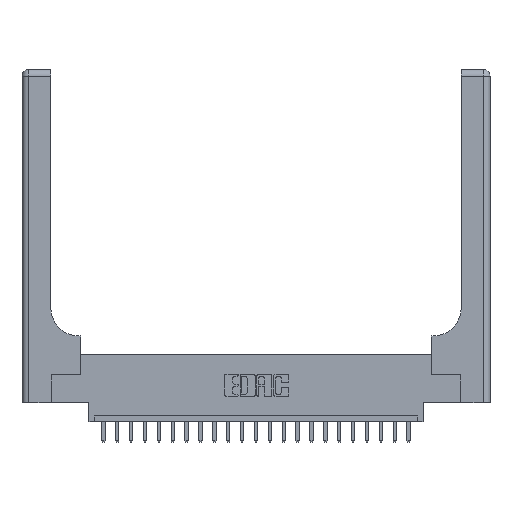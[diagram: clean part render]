
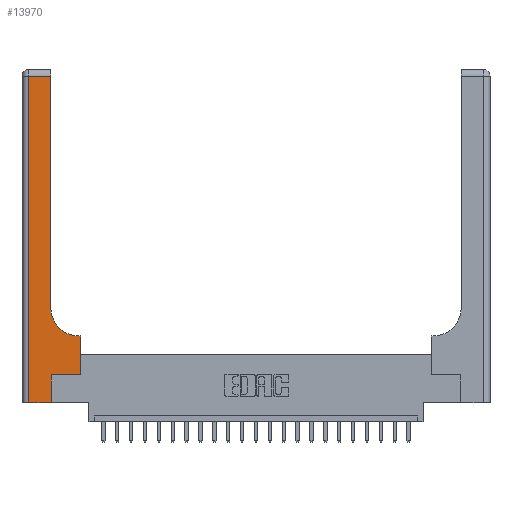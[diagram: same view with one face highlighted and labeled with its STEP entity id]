
A CAD part, top view. The second image highlights one B-rep face of the part: STEP entity #13970.
In plain terms, the highlighted planar face has unit normal (0, 0, 1).
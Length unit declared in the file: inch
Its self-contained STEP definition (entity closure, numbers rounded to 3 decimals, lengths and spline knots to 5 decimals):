
#11 = CARTESIAN_POINT ( 'NONE',  ( 0.26, 0.85, 0.37 ) ) ;
#16 = EDGE_CURVE ( 'NONE', #6308, #11377, #10593, .T. ) ;
#32 = CARTESIAN_POINT ( 'NONE',  ( 0.528, 0.25, 0.37 ) ) ;
#1361 = VECTOR ( 'NONE', #21693, 39.37008 ) ;
#1651 = CARTESIAN_POINT ( 'NONE',  ( 0.26, 2.94, 0.37 ) ) ;
#1661 = LINE ( 'NONE', #3941, #3279 ) ;
#2300 = VERTEX_POINT ( 'NONE', #7074 ) ;
#2553 = LINE ( 'NONE', #12259, #5292 ) ;
#3279 = VECTOR ( 'NONE', #16071, 39.37008 ) ;
#3343 = DIRECTION ( 'NONE',  ( 0., 0., -1. ) ) ;
#3627 = EDGE_CURVE ( 'NONE', #15931, #14777, #4854, .T. ) ;
#3761 = ORIENTED_EDGE ( 'NONE', *, *, #16470, .T. ) ;
#3941 = CARTESIAN_POINT ( 'NONE',  ( 0.26, 3., 0.37 ) ) ;
#4330 = CARTESIAN_POINT ( 'NONE',  ( 0.528, 0.25, 0.37 ) ) ;
#4854 = CIRCLE ( 'NONE', #6995, 0.25 ) ;
#5086 = ORIENTED_EDGE ( 'NONE', *, *, #20870, .T. ) ;
#5292 = VECTOR ( 'NONE', #6880, 39.37008 ) ;
#5703 = ORIENTED_EDGE ( 'NONE', *, *, #12226, .T. ) ;
#5906 = EDGE_CURVE ( 'NONE', #11377, #2300, #9012, .T. ) ;
#6043 = VECTOR ( 'NONE', #6108, 39.37008 ) ;
#6063 = DIRECTION ( 'NONE',  ( -1., 0., 0. ) ) ;
#6108 = DIRECTION ( 'NONE',  ( 1., 0., 0. ) ) ;
#6161 = VERTEX_POINT ( 'NONE', #18413 ) ;
#6300 = VECTOR ( 'NONE', #21127, 39.37008 ) ;
#6308 = VERTEX_POINT ( 'NONE', #6826 ) ;
#6321 = EDGE_LOOP ( 'NONE', ( #7735, #17940, #5086, #5703, #21645, #8040, #14710, #3761, #9540 ) ) ;
#6688 = VERTEX_POINT ( 'NONE', #16374 ) ;
#6826 = CARTESIAN_POINT ( 'NONE',  ( 0.265, 0.25, 0.37 ) ) ;
#6880 = DIRECTION ( 'NONE',  ( -1., 0., 0. ) ) ;
#6995 = AXIS2_PLACEMENT_3D ( 'NONE', #10307, #3343, #11828 ) ;
#7074 = CARTESIAN_POINT ( 'NONE',  ( 0.528, 0.6, 0.37 ) ) ;
#7302 = DIRECTION ( 'NONE',  ( 0., -1., 0. ) ) ;
#7735 = ORIENTED_EDGE ( 'NONE', *, *, #8329, .T. ) ;
#7770 = VECTOR ( 'NONE', #7302, 39.37008 ) ;
#7864 = CARTESIAN_POINT ( 'NONE',  ( 0., 2.94, 0.37 ) ) ;
#8009 = CARTESIAN_POINT ( 'NONE',  ( 0., 3., 0.37 ) ) ;
#8040 = ORIENTED_EDGE ( 'NONE', *, *, #16, .T. ) ;
#8329 = EDGE_CURVE ( 'NONE', #14777, #18326, #1661, .T. ) ;
#8909 = CARTESIAN_POINT ( 'NONE',  ( 0.06, 3., 0.37 ) ) ;
#9012 = LINE ( 'NONE', #32, #18676 ) ;
#9540 = ORIENTED_EDGE ( 'NONE', *, *, #3627, .T. ) ;
#10081 = DIRECTION ( 'NONE',  ( 0., 1., 0. ) ) ;
#10307 = CARTESIAN_POINT ( 'NONE',  ( 0.51, 0.85, 0.37 ) ) ;
#10593 = LINE ( 'NONE', #19721, #6043 ) ;
#11377 = VERTEX_POINT ( 'NONE', #4330 ) ;
#11828 = DIRECTION ( 'NONE',  ( 1., 0., 0. ) ) ;
#11845 = LINE ( 'NONE', #7864, #1361 ) ;
#11909 = VERTEX_POINT ( 'NONE', #16364 ) ;
#12057 = CARTESIAN_POINT ( 'NONE',  ( 0.51, 0.6, 0.37 ) ) ;
#12111 = VECTOR ( 'NONE', #13404, 39.37008 ) ;
#12226 = EDGE_CURVE ( 'NONE', #6161, #6688, #13014, .T. ) ;
#12259 = CARTESIAN_POINT ( 'NONE',  ( 0.26, 0.6, 0.37 ) ) ;
#13014 = LINE ( 'NONE', #18685, #6300 ) ;
#13260 = CARTESIAN_POINT ( 'NONE',  ( 0.265, 0., 0.37 ) ) ;
#13404 = DIRECTION ( 'NONE',  ( 0., 1., 0. ) ) ;
#13970 = ADVANCED_FACE ( 'NONE', ( #20150 ), #14819, .F. ) ;
#14029 = EDGE_CURVE ( 'NONE', #18326, #11909, #11845, .T. ) ;
#14107 = EDGE_CURVE ( 'NONE', #6688, #6308, #21245, .T. ) ;
#14710 = ORIENTED_EDGE ( 'NONE', *, *, #5906, .T. ) ;
#14777 = VERTEX_POINT ( 'NONE', #11 ) ;
#14819 = PLANE ( 'NONE',  #15699 ) ;
#15699 = AXIS2_PLACEMENT_3D ( 'NONE', #8009, #16542, #6063 ) ;
#15931 = VERTEX_POINT ( 'NONE', #12057 ) ;
#16071 = DIRECTION ( 'NONE',  ( 0., 1., 0. ) ) ;
#16094 = LINE ( 'NONE', #8909, #7770 ) ;
#16364 = CARTESIAN_POINT ( 'NONE',  ( 0.06, 2.94, 0.37 ) ) ;
#16374 = CARTESIAN_POINT ( 'NONE',  ( 0.265, 0., 0.37 ) ) ;
#16470 = EDGE_CURVE ( 'NONE', #2300, #15931, #2553, .T. ) ;
#16542 = DIRECTION ( 'NONE',  ( 0., 0., -1. ) ) ;
#17940 = ORIENTED_EDGE ( 'NONE', *, *, #14029, .T. ) ;
#18326 = VERTEX_POINT ( 'NONE', #1651 ) ;
#18413 = CARTESIAN_POINT ( 'NONE',  ( 0.06, 0., 0.37 ) ) ;
#18676 = VECTOR ( 'NONE', #10081, 39.37008 ) ;
#18685 = CARTESIAN_POINT ( 'NONE',  ( 0., 0., 0.37 ) ) ;
#19721 = CARTESIAN_POINT ( 'NONE',  ( 0.265, 0.25, 0.37 ) ) ;
#20150 = FACE_OUTER_BOUND ( 'NONE', #6321, .T. ) ;
#20870 = EDGE_CURVE ( 'NONE', #11909, #6161, #16094, .T. ) ;
#21127 = DIRECTION ( 'NONE',  ( 1., 0., 0. ) ) ;
#21245 = LINE ( 'NONE', #13260, #12111 ) ;
#21645 = ORIENTED_EDGE ( 'NONE', *, *, #14107, .T. ) ;
#21693 = DIRECTION ( 'NONE',  ( -1., 0., 0. ) ) ;
